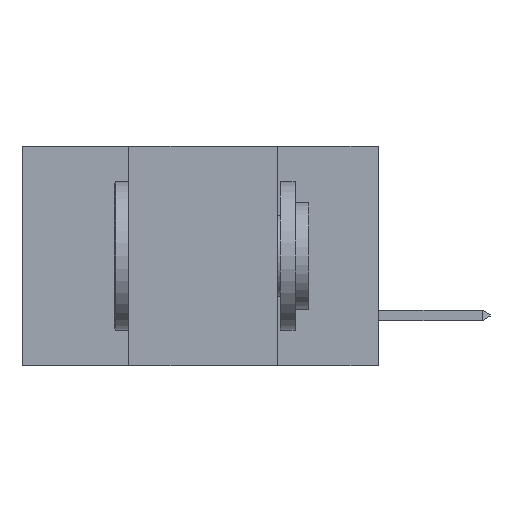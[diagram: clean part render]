
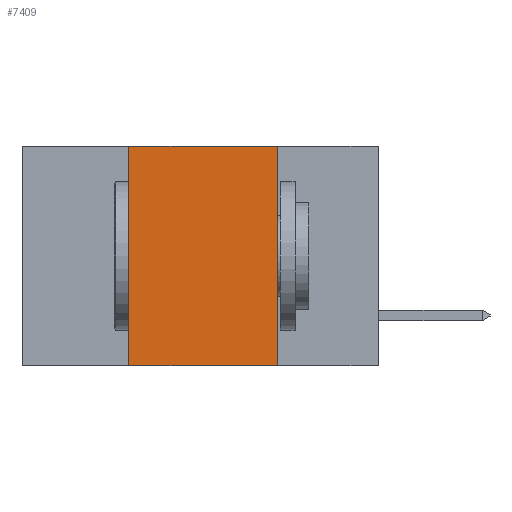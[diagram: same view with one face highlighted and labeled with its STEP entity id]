
A CAD part, left-side view. The second image highlights one B-rep face of the part: STEP entity #7409.
In plain terms, the highlighted planar face has unit normal (-1, 0, 0).
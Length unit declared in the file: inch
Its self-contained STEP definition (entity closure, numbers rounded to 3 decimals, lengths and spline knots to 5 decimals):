
#51 = DIRECTION ( 'NONE',  ( 0., 0., 1. ) ) ;
#962 = DIRECTION ( 'NONE',  ( 0., -1., 0. ) ) ;
#1550 = FACE_OUTER_BOUND ( 'NONE', #26240, .T. ) ;
#1667 = VECTOR ( 'NONE', #7956, 39.37008 ) ;
#2139 = DIRECTION ( 'NONE',  ( 1., 0., 0. ) ) ;
#3297 = ORIENTED_EDGE ( 'NONE', *, *, #25056, .F. ) ;
#4120 = ORIENTED_EDGE ( 'NONE', *, *, #6133, .F. ) ;
#4777 = CARTESIAN_POINT ( 'NONE',  ( 0., 0.42, 0. ) ) ;
#5466 = VERTEX_POINT ( 'NONE', #14856 ) ;
#5937 = VECTOR ( 'NONE', #962, 39.37008 ) ;
#6133 = EDGE_CURVE ( 'NONE', #21242, #23378, #23693, .T. ) ;
#7229 = LINE ( 'NONE', #8044, #1667 ) ;
#7409 = ADVANCED_FACE ( 'NONE', ( #1550 ), #10479, .F. ) ;
#7956 = DIRECTION ( 'NONE',  ( 0., 0., -1. ) ) ;
#8044 = CARTESIAN_POINT ( 'NONE',  ( 0., 0.17, 0. ) ) ;
#8355 = VERTEX_POINT ( 'NONE', #20630 ) ;
#8682 = ORIENTED_EDGE ( 'NONE', *, *, #12678, .T. ) ;
#10479 = PLANE ( 'NONE',  #20731 ) ;
#11440 = CARTESIAN_POINT ( 'NONE',  ( 0., 0.6, 0. ) ) ;
#12678 = EDGE_CURVE ( 'NONE', #21242, #8355, #22837, .T. ) ;
#12986 = VECTOR ( 'NONE', #51, 39.37008 ) ;
#14678 = CARTESIAN_POINT ( 'NONE',  ( 0., 0.6, 0. ) ) ;
#14856 = CARTESIAN_POINT ( 'NONE',  ( 0., 0.17, 0. ) ) ;
#15298 = DIRECTION ( 'NONE',  ( 0., -1., 0. ) ) ;
#16725 = DIRECTION ( 'NONE',  ( 0., 0., -1. ) ) ;
#17197 = EDGE_CURVE ( 'NONE', #23378, #5466, #17650, .T. ) ;
#17249 = VECTOR ( 'NONE', #15298, 39.37008 ) ;
#17650 = LINE ( 'NONE', #11440, #5937 ) ;
#20630 = CARTESIAN_POINT ( 'NONE',  ( 0., 0.17, -0.37 ) ) ;
#20731 = AXIS2_PLACEMENT_3D ( 'NONE', #14678, #2139, #16725 ) ;
#21242 = VERTEX_POINT ( 'NONE', #23627 ) ;
#21266 = CARTESIAN_POINT ( 'NONE',  ( 0., 0.6, -0.37 ) ) ;
#22837 = LINE ( 'NONE', #21266, #17249 ) ;
#22986 = ORIENTED_EDGE ( 'NONE', *, *, #17197, .F. ) ;
#23378 = VERTEX_POINT ( 'NONE', #4777 ) ;
#23627 = CARTESIAN_POINT ( 'NONE',  ( 0., 0.42, -0.37 ) ) ;
#23693 = LINE ( 'NONE', #24716, #12986 ) ;
#24716 = CARTESIAN_POINT ( 'NONE',  ( 0., 0.42, 0. ) ) ;
#25056 = EDGE_CURVE ( 'NONE', #5466, #8355, #7229, .T. ) ;
#26240 = EDGE_LOOP ( 'NONE', ( #3297, #22986, #4120, #8682 ) ) ;
